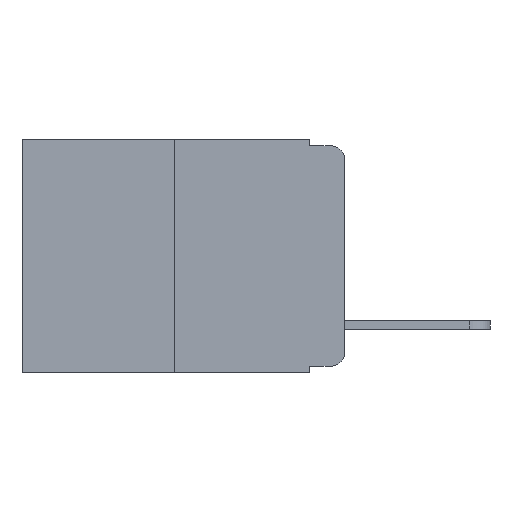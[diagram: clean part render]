
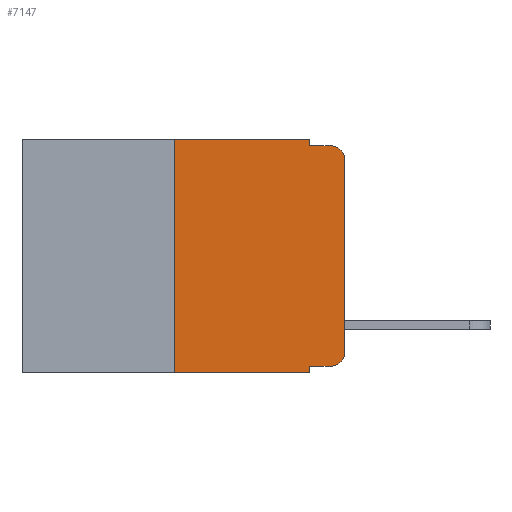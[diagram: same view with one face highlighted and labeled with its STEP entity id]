
A CAD part, left-side view. The second image highlights one B-rep face of the part: STEP entity #7147.
In plain terms, the highlighted planar face has unit normal (-1, 0, 0).
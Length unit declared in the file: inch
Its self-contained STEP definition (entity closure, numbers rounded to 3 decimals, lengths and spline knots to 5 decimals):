
#86 = EDGE_CURVE ( 'NONE', #10116, #3997, #8148, .T. ) ;
#196 = ORIENTED_EDGE ( 'NONE', *, *, #86, .T. ) ;
#628 = EDGE_CURVE ( 'NONE', #1842, #7971, #4552, .T. ) ;
#661 = ORIENTED_EDGE ( 'NONE', *, *, #3640, .F. ) ;
#679 = DIRECTION ( 'NONE',  ( 0., 0., -1. ) ) ;
#1155 = VERTEX_POINT ( 'NONE', #12500 ) ;
#1504 = DIRECTION ( 'NONE',  ( -1., 0., 0. ) ) ;
#1654 = DIRECTION ( 'NONE',  ( 0., 0., 1. ) ) ;
#1842 = VERTEX_POINT ( 'NONE', #14771 ) ;
#2120 = LINE ( 'NONE', #12590, #11323 ) ;
#2251 = EDGE_CURVE ( 'NONE', #12071, #1842, #2120, .T. ) ;
#2276 = CARTESIAN_POINT ( 'NONE',  ( 0., 0.473, 0. ) ) ;
#3078 = FACE_OUTER_BOUND ( 'NONE', #14930, .T. ) ;
#3133 = DIRECTION ( 'NONE',  ( 0., 0., -1. ) ) ;
#3509 = LINE ( 'NONE', #15281, #7052 ) ;
#3562 = DIRECTION ( 'NONE',  ( 0., 0., -1. ) ) ;
#3640 = EDGE_CURVE ( 'NONE', #7971, #11892, #6730, .T. ) ;
#3880 = CARTESIAN_POINT ( 'NONE',  ( 0., 0.02, -0.313 ) ) ;
#3997 = VERTEX_POINT ( 'NONE', #10728 ) ;
#4043 = DIRECTION ( 'NONE',  ( 0., -1., 0. ) ) ;
#4232 = EDGE_CURVE ( 'NONE', #15515, #1155, #11403, .T. ) ;
#4552 = LINE ( 'NONE', #5420, #10576 ) ;
#4565 = DIRECTION ( 'NONE',  ( 0., -1., 0. ) ) ;
#4583 = AXIS2_PLACEMENT_3D ( 'NONE', #5411, #15011, #3562 ) ;
#5371 = ORIENTED_EDGE ( 'NONE', *, *, #13276, .F. ) ;
#5411 = CARTESIAN_POINT ( 'NONE',  ( 0., 0.02, -0.03 ) ) ;
#5420 = CARTESIAN_POINT ( 'NONE',  ( 0., 0.473, 0. ) ) ;
#5724 = CARTESIAN_POINT ( 'NONE',  ( 0., 0.473, -0.343 ) ) ;
#5970 = EDGE_CURVE ( 'NONE', #12071, #13495, #15474, .T. ) ;
#6132 = LINE ( 'NONE', #11240, #9712 ) ;
#6381 = ORIENTED_EDGE ( 'NONE', *, *, #12583, .T. ) ;
#6496 = ORIENTED_EDGE ( 'NONE', *, *, #2251, .F. ) ;
#6730 = LINE ( 'NONE', #7979, #11262 ) ;
#6842 = LINE ( 'NONE', #14128, #7221 ) ;
#6875 = CARTESIAN_POINT ( 'NONE',  ( 0., 0.051, 0. ) ) ;
#6961 = PLANE ( 'NONE',  #12546 ) ;
#7052 = VECTOR ( 'NONE', #12849, 39.37008 ) ;
#7147 = ADVANCED_FACE ( 'NONE', ( #3078 ), #6961, .F. ) ;
#7221 = VECTOR ( 'NONE', #4565, 39.37008 ) ;
#7322 = LINE ( 'NONE', #13973, #12960 ) ;
#7798 = ORIENTED_EDGE ( 'NONE', *, *, #12306, .T. ) ;
#7960 = CARTESIAN_POINT ( 'NONE',  ( 0., 0.051, -0.333 ) ) ;
#7971 = VERTEX_POINT ( 'NONE', #6875 ) ;
#7979 = CARTESIAN_POINT ( 'NONE',  ( 0., 0.051, 0. ) ) ;
#8148 = CIRCLE ( 'NONE', #9462, 0.02 ) ;
#8719 = DIRECTION ( 'NONE',  ( 0., 0., -1. ) ) ;
#9346 = ORIENTED_EDGE ( 'NONE', *, *, #10667, .F. ) ;
#9391 = DIRECTION ( 'NONE',  ( 1., 0., 0. ) ) ;
#9462 = AXIS2_PLACEMENT_3D ( 'NONE', #3880, #1504, #8719 ) ;
#9670 = VECTOR ( 'NONE', #10511, 39.37008 ) ;
#9712 = VECTOR ( 'NONE', #4043, 39.37008 ) ;
#10116 = VERTEX_POINT ( 'NONE', #14550 ) ;
#10147 = CARTESIAN_POINT ( 'NONE',  ( 0., 0., -0.03 ) ) ;
#10511 = DIRECTION ( 'NONE',  ( 0., -1., 0. ) ) ;
#10576 = VECTOR ( 'NONE', #13821, 39.37008 ) ;
#10593 = DIRECTION ( 'NONE',  ( 0., 0., -1. ) ) ;
#10667 = EDGE_CURVE ( 'NONE', #15056, #13495, #7322, .T. ) ;
#10728 = CARTESIAN_POINT ( 'NONE',  ( 0., 0., -0.313 ) ) ;
#11240 = CARTESIAN_POINT ( 'NONE',  ( 0., 0.051, -0.333 ) ) ;
#11262 = VECTOR ( 'NONE', #679, 39.37008 ) ;
#11323 = VECTOR ( 'NONE', #1654, 39.37008 ) ;
#11403 = CIRCLE ( 'NONE', #4583, 0.02 ) ;
#11892 = VERTEX_POINT ( 'NONE', #12369 ) ;
#11935 = CARTESIAN_POINT ( 'NONE',  ( 0., 0.25, -0.343 ) ) ;
#12071 = VERTEX_POINT ( 'NONE', #11935 ) ;
#12306 = EDGE_CURVE ( 'NONE', #15056, #10116, #6132, .T. ) ;
#12369 = CARTESIAN_POINT ( 'NONE',  ( 0., 0.051, -0.01 ) ) ;
#12500 = CARTESIAN_POINT ( 'NONE',  ( 0., 0.02, -0.01 ) ) ;
#12546 = AXIS2_PLACEMENT_3D ( 'NONE', #2276, #9391, #10593 ) ;
#12583 = EDGE_CURVE ( 'NONE', #3997, #15515, #3509, .T. ) ;
#12590 = CARTESIAN_POINT ( 'NONE',  ( 0., 0.25, 0. ) ) ;
#12794 = ORIENTED_EDGE ( 'NONE', *, *, #4232, .T. ) ;
#12849 = DIRECTION ( 'NONE',  ( 0., 0., 1. ) ) ;
#12960 = VECTOR ( 'NONE', #3133, 39.37008 ) ;
#13276 = EDGE_CURVE ( 'NONE', #11892, #1155, #6842, .T. ) ;
#13495 = VERTEX_POINT ( 'NONE', #13892 ) ;
#13653 = ORIENTED_EDGE ( 'NONE', *, *, #5970, .T. ) ;
#13821 = DIRECTION ( 'NONE',  ( 0., -1., 0. ) ) ;
#13892 = CARTESIAN_POINT ( 'NONE',  ( 0., 0.051, -0.343 ) ) ;
#13973 = CARTESIAN_POINT ( 'NONE',  ( 0., 0.051, 0. ) ) ;
#14128 = CARTESIAN_POINT ( 'NONE',  ( 0., 0.051, -0.01 ) ) ;
#14550 = CARTESIAN_POINT ( 'NONE',  ( 0., 0.02, -0.333 ) ) ;
#14771 = CARTESIAN_POINT ( 'NONE',  ( 0., 0.25, 0. ) ) ;
#14930 = EDGE_LOOP ( 'NONE', ( #6381, #12794, #5371, #661, #14967, #6496, #13653, #9346, #7798, #196 ) ) ;
#14967 = ORIENTED_EDGE ( 'NONE', *, *, #628, .F. ) ;
#15011 = DIRECTION ( 'NONE',  ( -1., 0., 0. ) ) ;
#15056 = VERTEX_POINT ( 'NONE', #7960 ) ;
#15281 = CARTESIAN_POINT ( 'NONE',  ( 0., 0., 0. ) ) ;
#15474 = LINE ( 'NONE', #5724, #9670 ) ;
#15515 = VERTEX_POINT ( 'NONE', #10147 ) ;
